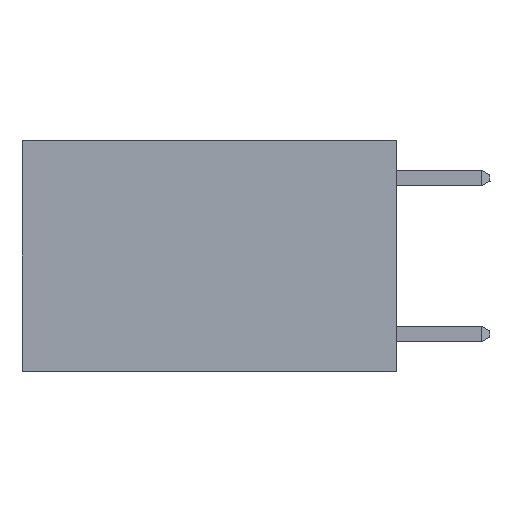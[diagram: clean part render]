
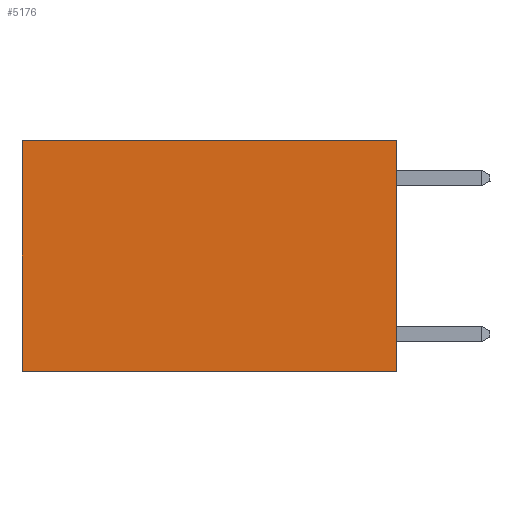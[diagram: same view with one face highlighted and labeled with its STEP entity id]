
A CAD part, left-side view. The second image highlights one B-rep face of the part: STEP entity #5176.
In plain terms, the highlighted planar face has unit normal (-1, 0, 0).
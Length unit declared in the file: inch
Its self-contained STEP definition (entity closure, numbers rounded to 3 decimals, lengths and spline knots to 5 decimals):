
#109 = CARTESIAN_POINT ( 'NONE',  ( 0.2625, 0.6, 0. ) ) ;
#173 = VERTEX_POINT ( 'NONE', #1431 ) ;
#234 = DIRECTION ( 'NONE',  ( 1., 0., 0. ) ) ;
#239 = VERTEX_POINT ( 'NONE', #5672 ) ;
#278 = VECTOR ( 'NONE', #2235, 39.37008 ) ;
#334 = ORIENTED_EDGE ( 'NONE', *, *, #3392, .T. ) ;
#520 = LINE ( 'NONE', #109, #3216 ) ;
#854 = VECTOR ( 'NONE', #2155, 39.37008 ) ;
#1291 = VECTOR ( 'NONE', #4072, 39.37008 ) ;
#1383 = LINE ( 'NONE', #8399, #1291 ) ;
#1431 = CARTESIAN_POINT ( 'NONE',  ( 0.2625, 0., -0.37 ) ) ;
#1911 = ORIENTED_EDGE ( 'NONE', *, *, #4633, .T. ) ;
#2155 = DIRECTION ( 'NONE',  ( 0., 0., -1. ) ) ;
#2214 = CARTESIAN_POINT ( 'NONE',  ( 0.2625, 0., 0. ) ) ;
#2235 = DIRECTION ( 'NONE',  ( 0., 1., 0. ) ) ;
#2258 = CARTESIAN_POINT ( 'NONE',  ( 0.2625, 0.6, -0.37 ) ) ;
#3099 = VERTEX_POINT ( 'NONE', #2258 ) ;
#3216 = VECTOR ( 'NONE', #4478, 39.37008 ) ;
#3325 = PLANE ( 'NONE',  #4919 ) ;
#3392 = EDGE_CURVE ( 'NONE', #239, #3099, #520, .T. ) ;
#3395 = VERTEX_POINT ( 'NONE', #2214 ) ;
#3444 = EDGE_LOOP ( 'NONE', ( #334, #4983, #8218, #1911 ) ) ;
#3445 = EDGE_CURVE ( 'NONE', #3395, #173, #4389, .T. ) ;
#4072 = DIRECTION ( 'NONE',  ( 0., 1., 0. ) ) ;
#4389 = LINE ( 'NONE', #6851, #854 ) ;
#4478 = DIRECTION ( 'NONE',  ( 0., 0., -1. ) ) ;
#4597 = FACE_OUTER_BOUND ( 'NONE', #3444, .T. ) ;
#4633 = EDGE_CURVE ( 'NONE', #3395, #239, #1383, .T. ) ;
#4886 = CARTESIAN_POINT ( 'NONE',  ( 0.2625, 0., -0.37 ) ) ;
#4919 = AXIS2_PLACEMENT_3D ( 'NONE', #6991, #234, #5065 ) ;
#4983 = ORIENTED_EDGE ( 'NONE', *, *, #7531, .F. ) ;
#5065 = DIRECTION ( 'NONE',  ( 0., 0., -1. ) ) ;
#5172 = LINE ( 'NONE', #4886, #278 ) ;
#5176 = ADVANCED_FACE ( 'NONE', ( #4597 ), #3325, .F. ) ;
#5672 = CARTESIAN_POINT ( 'NONE',  ( 0.2625, 0.6, 0. ) ) ;
#6851 = CARTESIAN_POINT ( 'NONE',  ( 0.2625, 0., 0. ) ) ;
#6991 = CARTESIAN_POINT ( 'NONE',  ( 0.2625, 0., 0. ) ) ;
#7531 = EDGE_CURVE ( 'NONE', #173, #3099, #5172, .T. ) ;
#8218 = ORIENTED_EDGE ( 'NONE', *, *, #3445, .F. ) ;
#8399 = CARTESIAN_POINT ( 'NONE',  ( 0.2625, 0., 0. ) ) ;
